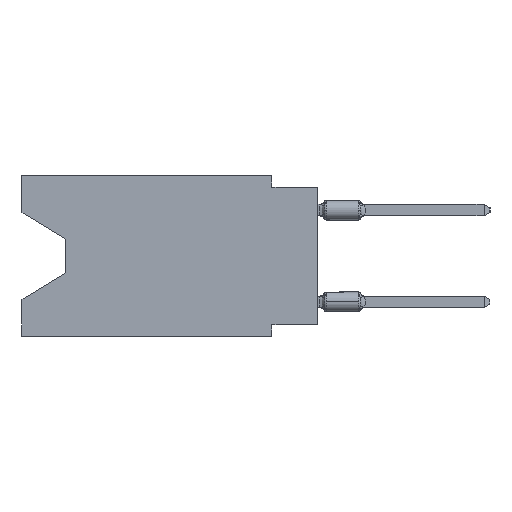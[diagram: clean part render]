
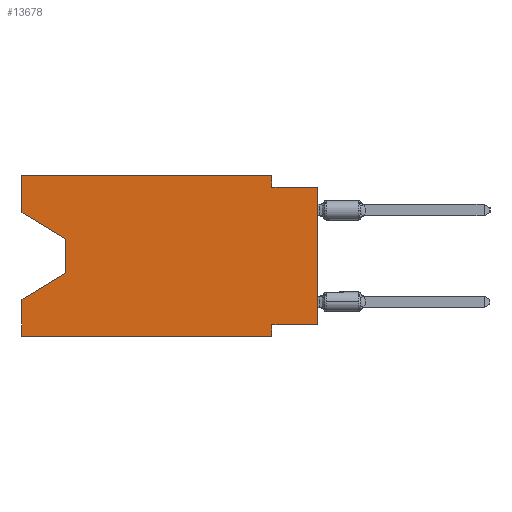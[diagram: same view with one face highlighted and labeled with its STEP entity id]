
A CAD part, left-side view. The second image highlights one B-rep face of the part: STEP entity #13678.
In plain terms, the highlighted planar face has unit normal (-1, 0, 0).
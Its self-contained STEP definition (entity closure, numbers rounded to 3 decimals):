
#244 = CARTESIAN_POINT ( 'NONE',  ( 0., 16.383, -8.89 ) ) ;
#713 = EDGE_CURVE ( 'NONE', #22245, #16359, #7381, .T. ) ;
#964 = EDGE_CURVE ( 'NONE', #16050, #16359, #26365, .T. ) ;
#1921 = EDGE_CURVE ( 'NONE', #27843, #3329, #3822, .T. ) ;
#2363 = LINE ( 'NONE', #244, #7812 ) ;
#3004 = DIRECTION ( 'NONE',  ( 0., 0.855, -0.519 ) ) ;
#3211 = VERTEX_POINT ( 'NONE', #21862 ) ;
#3329 = VERTEX_POINT ( 'NONE', #24641 ) ;
#3815 = VERTEX_POINT ( 'NONE', #18712 ) ;
#3822 = LINE ( 'NONE', #27751, #13508 ) ;
#3868 = VERTEX_POINT ( 'NONE', #13535 ) ;
#3948 = EDGE_LOOP ( 'NONE', ( #17408, #6152, #19612, #10356, #4102, #23685, #11690, #10410, #11597, #21768, #20153, #18175 ) ) ;
#4102 = ORIENTED_EDGE ( 'NONE', *, *, #23005, .T. ) ;
#4148 = DIRECTION ( 'NONE',  ( 0., -1., 0. ) ) ;
#4326 = CARTESIAN_POINT ( 'NONE',  ( 0., 13.97, -3.505 ) ) ;
#5739 = CARTESIAN_POINT ( 'NONE',  ( 0., 2.54, -8.255 ) ) ;
#5965 = LINE ( 'NONE', #16524, #14891 ) ;
#6152 = ORIENTED_EDGE ( 'NONE', *, *, #24561, .T. ) ;
#6876 = VECTOR ( 'NONE', #14612, 1000. ) ;
#7381 = LINE ( 'NONE', #14278, #27856 ) ;
#7748 = VECTOR ( 'NONE', #3004, 1000. ) ;
#7812 = VECTOR ( 'NONE', #8558, 1000. ) ;
#8154 = EDGE_CURVE ( 'NONE', #3211, #3815, #13735, .T. ) ;
#8339 = FACE_OUTER_BOUND ( 'NONE', #3948, .T. ) ;
#8501 = LINE ( 'NONE', #23589, #23512 ) ;
#8558 = DIRECTION ( 'NONE',  ( 0., -1., 0. ) ) ;
#8697 = DIRECTION ( 'NONE',  ( 0., 0., -1. ) ) ;
#8699 = CARTESIAN_POINT ( 'NONE',  ( 0., 16.383, 0. ) ) ;
#8933 = EDGE_CURVE ( 'NONE', #16050, #26628, #26560, .T. ) ;
#8957 = EDGE_CURVE ( 'NONE', #20383, #22245, #19980, .T. ) ;
#9089 = EDGE_CURVE ( 'NONE', #26628, #3868, #23054, .T. ) ;
#10165 = DIRECTION ( 'NONE',  ( 0., -0.855, -0.519 ) ) ;
#10356 = ORIENTED_EDGE ( 'NONE', *, *, #26360, .F. ) ;
#10410 = ORIENTED_EDGE ( 'NONE', *, *, #964, .T. ) ;
#10454 = DIRECTION ( 'NONE',  ( 0., 0., -1. ) ) ;
#10485 = VECTOR ( 'NONE', #17856, 1000. ) ;
#10758 = CARTESIAN_POINT ( 'NONE',  ( 0., 16.383, 0. ) ) ;
#10801 = EDGE_CURVE ( 'NONE', #25517, #20383, #8501, .T. ) ;
#11597 = ORIENTED_EDGE ( 'NONE', *, *, #713, .F. ) ;
#11644 = CARTESIAN_POINT ( 'NONE',  ( 0., 2.54, 0. ) ) ;
#11690 = ORIENTED_EDGE ( 'NONE', *, *, #8933, .F. ) ;
#12364 = CARTESIAN_POINT ( 'NONE',  ( 0., 2.54, -8.89 ) ) ;
#13340 = EDGE_CURVE ( 'NONE', #27843, #25517, #21601, .T. ) ;
#13466 = VECTOR ( 'NONE', #15548, 1000. ) ;
#13488 = DIRECTION ( 'NONE',  ( 0., 1., 0. ) ) ;
#13508 = VECTOR ( 'NONE', #10165, 1000. ) ;
#13535 = CARTESIAN_POINT ( 'NONE',  ( 0., 2.54, -8.89 ) ) ;
#13678 = ADVANCED_FACE ( 'NONE', ( #8339 ), #25928, .F. ) ;
#13735 = LINE ( 'NONE', #22316, #7748 ) ;
#14278 = CARTESIAN_POINT ( 'NONE',  ( 0., 0., -0.635 ) ) ;
#14612 = DIRECTION ( 'NONE',  ( 0., 0., -1. ) ) ;
#14891 = VECTOR ( 'NONE', #23415, 1000. ) ;
#15548 = DIRECTION ( 'NONE',  ( 0., 0., 1. ) ) ;
#16050 = VERTEX_POINT ( 'NONE', #18412 ) ;
#16359 = VERTEX_POINT ( 'NONE', #16385 ) ;
#16385 = CARTESIAN_POINT ( 'NONE',  ( 0., 0., -0.635 ) ) ;
#16524 = CARTESIAN_POINT ( 'NONE',  ( 0., 16.383, 0. ) ) ;
#17195 = CARTESIAN_POINT ( 'NONE',  ( 0., 16.383, -2.038 ) ) ;
#17408 = ORIENTED_EDGE ( 'NONE', *, *, #1921, .T. ) ;
#17856 = DIRECTION ( 'NONE',  ( 0., 0., -1. ) ) ;
#18175 = ORIENTED_EDGE ( 'NONE', *, *, #13340, .F. ) ;
#18412 = CARTESIAN_POINT ( 'NONE',  ( 0., 0., -8.255 ) ) ;
#18472 = CARTESIAN_POINT ( 'NONE',  ( 0., 2.54, -0.635 ) ) ;
#18712 = CARTESIAN_POINT ( 'NONE',  ( 0., 16.383, -6.852 ) ) ;
#19612 = ORIENTED_EDGE ( 'NONE', *, *, #8154, .T. ) ;
#19980 = LINE ( 'NONE', #11644, #10485 ) ;
#20153 = ORIENTED_EDGE ( 'NONE', *, *, #10801, .F. ) ;
#20362 = VECTOR ( 'NONE', #13488, 1000. ) ;
#20383 = VERTEX_POINT ( 'NONE', #21900 ) ;
#21559 = VECTOR ( 'NONE', #8697, 1000. ) ;
#21590 = CARTESIAN_POINT ( 'NONE',  ( 0., 0., 0. ) ) ;
#21601 = LINE ( 'NONE', #10758, #22299 ) ;
#21768 = ORIENTED_EDGE ( 'NONE', *, *, #8957, .F. ) ;
#21862 = CARTESIAN_POINT ( 'NONE',  ( 0., 13.97, -5.385 ) ) ;
#21900 = CARTESIAN_POINT ( 'NONE',  ( 0., 2.54, 0. ) ) ;
#21994 = CARTESIAN_POINT ( 'NONE',  ( 0., 16.383, -8.89 ) ) ;
#22245 = VERTEX_POINT ( 'NONE', #18472 ) ;
#22299 = VECTOR ( 'NONE', #23434, 1000. ) ;
#22316 = CARTESIAN_POINT ( 'NONE',  ( 0., 13.97, -5.385 ) ) ;
#22858 = DIRECTION ( 'NONE',  ( 0., -1., 0. ) ) ;
#23005 = EDGE_CURVE ( 'NONE', #26606, #3868, #2363, .T. ) ;
#23054 = LINE ( 'NONE', #12364, #6876 ) ;
#23415 = DIRECTION ( 'NONE',  ( 0., 0., 1. ) ) ;
#23434 = DIRECTION ( 'NONE',  ( 0., 0., 1. ) ) ;
#23512 = VECTOR ( 'NONE', #4148, 1000. ) ;
#23589 = CARTESIAN_POINT ( 'NONE',  ( 0., 16.383, 0. ) ) ;
#23685 = ORIENTED_EDGE ( 'NONE', *, *, #9089, .F. ) ;
#24464 = CARTESIAN_POINT ( 'NONE',  ( 0., 0., -8.255 ) ) ;
#24480 = CARTESIAN_POINT ( 'NONE',  ( 0., 16.383, 0. ) ) ;
#24561 = EDGE_CURVE ( 'NONE', #3329, #3211, #25726, .T. ) ;
#24641 = CARTESIAN_POINT ( 'NONE',  ( 0., 13.97, -3.505 ) ) ;
#25505 = DIRECTION ( 'NONE',  ( 1., 0., 0. ) ) ;
#25517 = VERTEX_POINT ( 'NONE', #24480 ) ;
#25726 = LINE ( 'NONE', #4326, #21559 ) ;
#25928 = PLANE ( 'NONE',  #27266 ) ;
#26360 = EDGE_CURVE ( 'NONE', #26606, #3815, #5965, .T. ) ;
#26365 = LINE ( 'NONE', #21590, #13466 ) ;
#26560 = LINE ( 'NONE', #24464, #20362 ) ;
#26606 = VERTEX_POINT ( 'NONE', #21994 ) ;
#26628 = VERTEX_POINT ( 'NONE', #5739 ) ;
#27266 = AXIS2_PLACEMENT_3D ( 'NONE', #8699, #25505, #10454 ) ;
#27751 = CARTESIAN_POINT ( 'NONE',  ( 0., 16.383, -2.038 ) ) ;
#27843 = VERTEX_POINT ( 'NONE', #17195 ) ;
#27856 = VECTOR ( 'NONE', #22858, 1000. ) ;
